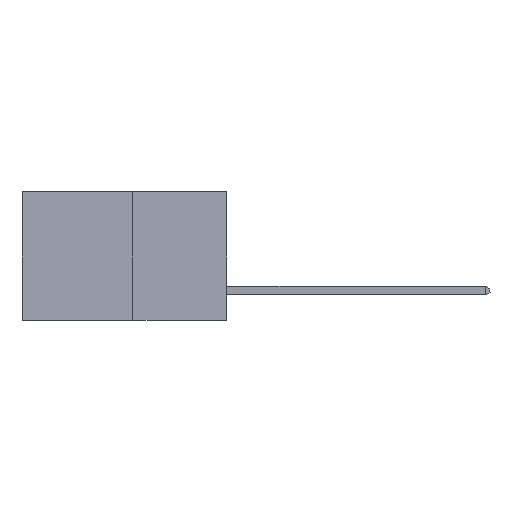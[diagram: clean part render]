
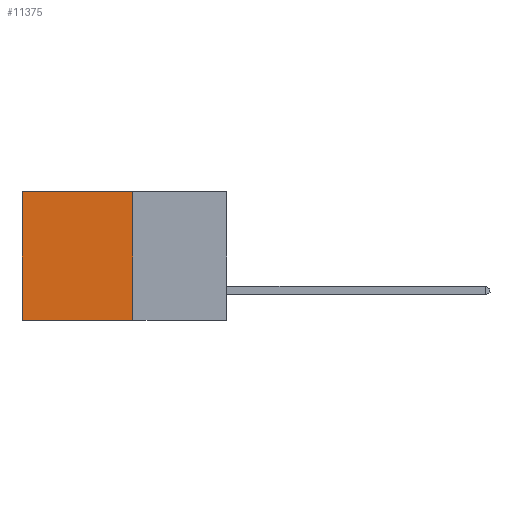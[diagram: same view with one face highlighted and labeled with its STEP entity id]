
A CAD part, left-side view. The second image highlights one B-rep face of the part: STEP entity #11375.
In plain terms, the highlighted planar face has unit normal (-1, 0, 0).
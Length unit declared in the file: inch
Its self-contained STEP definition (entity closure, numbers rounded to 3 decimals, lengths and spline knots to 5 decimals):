
#164 = DIRECTION ( 'NONE',  ( 0., 1., 0. ) ) ;
#265 = EDGE_CURVE ( 'NONE', #2693, #12348, #11697, .T. ) ;
#723 = ORIENTED_EDGE ( 'NONE', *, *, #2153, .F. ) ;
#892 = EDGE_CURVE ( 'NONE', #12348, #12289, #13010, .T. ) ;
#1201 = EDGE_CURVE ( 'NONE', #4897, #12289, #9810, .T. ) ;
#1235 = DIRECTION ( 'NONE',  ( 0., 0., -1. ) ) ;
#2153 = EDGE_CURVE ( 'NONE', #2693, #4897, #3177, .T. ) ;
#2690 = VECTOR ( 'NONE', #3159, 39.37008 ) ;
#2693 = VERTEX_POINT ( 'NONE', #8390 ) ;
#2813 = VECTOR ( 'NONE', #1235, 39.37008 ) ;
#3159 = DIRECTION ( 'NONE',  ( 0., 0., -1. ) ) ;
#3177 = LINE ( 'NONE', #10187, #2813 ) ;
#3387 = PLANE ( 'NONE',  #12128 ) ;
#3607 = ORIENTED_EDGE ( 'NONE', *, *, #1201, .F. ) ;
#4389 = VECTOR ( 'NONE', #164, 39.37008 ) ;
#4563 = CARTESIAN_POINT ( 'NONE',  ( 0.277, 0.27, -0.37 ) ) ;
#4586 = DIRECTION ( 'NONE',  ( 1., 0., 0. ) ) ;
#4897 = VERTEX_POINT ( 'NONE', #12718 ) ;
#5637 = ORIENTED_EDGE ( 'NONE', *, *, #265, .T. ) ;
#6417 = CARTESIAN_POINT ( 'NONE',  ( 0.277, 0.59, 0. ) ) ;
#7969 = DIRECTION ( 'NONE',  ( 0., 1., 0. ) ) ;
#8190 = EDGE_LOOP ( 'NONE', ( #12607, #3607, #723, #5637 ) ) ;
#8390 = CARTESIAN_POINT ( 'NONE',  ( 0.277, 0.27, 0. ) ) ;
#9810 = LINE ( 'NONE', #4563, #4389 ) ;
#10187 = CARTESIAN_POINT ( 'NONE',  ( 0.277, 0.27, -0.37 ) ) ;
#10318 = CARTESIAN_POINT ( 'NONE',  ( 0.277, 0.27, -0.37 ) ) ;
#10561 = FACE_OUTER_BOUND ( 'NONE', #8190, .T. ) ;
#11035 = CARTESIAN_POINT ( 'NONE',  ( 0.277, 0.59, -0.37 ) ) ;
#11229 = DIRECTION ( 'NONE',  ( 0., 0., -1. ) ) ;
#11316 = CARTESIAN_POINT ( 'NONE',  ( 0.277, 0.27, 0. ) ) ;
#11375 = ADVANCED_FACE ( 'NONE', ( #10561 ), #3387, .F. ) ;
#11430 = VECTOR ( 'NONE', #7969, 39.37008 ) ;
#11697 = LINE ( 'NONE', #11316, #11430 ) ;
#12128 = AXIS2_PLACEMENT_3D ( 'NONE', #10318, #4586, #11229 ) ;
#12289 = VERTEX_POINT ( 'NONE', #11035 ) ;
#12348 = VERTEX_POINT ( 'NONE', #6417 ) ;
#12607 = ORIENTED_EDGE ( 'NONE', *, *, #892, .T. ) ;
#12718 = CARTESIAN_POINT ( 'NONE',  ( 0.277, 0.27, -0.37 ) ) ;
#12860 = CARTESIAN_POINT ( 'NONE',  ( 0.277, 0.59, -0.37 ) ) ;
#13010 = LINE ( 'NONE', #12860, #2690 ) ;
